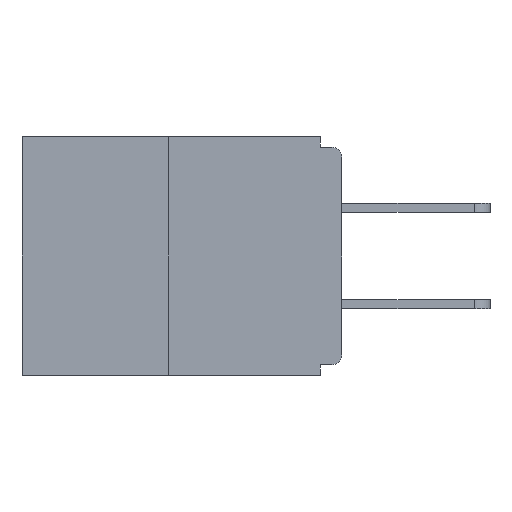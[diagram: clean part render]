
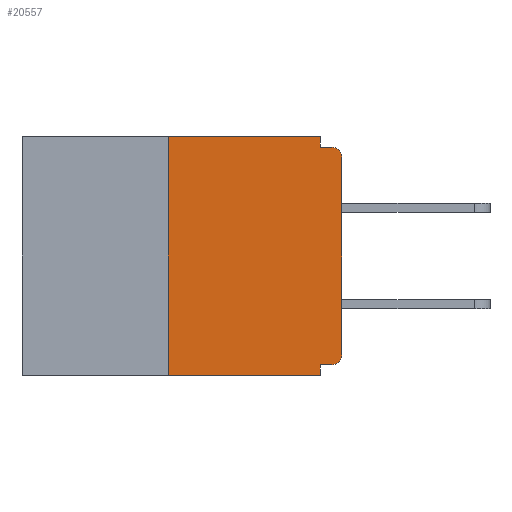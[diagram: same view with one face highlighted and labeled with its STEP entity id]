
A CAD part, left-side view. The second image highlights one B-rep face of the part: STEP entity #20557.
In plain terms, the highlighted planar face has unit normal (-1, 0, 0).
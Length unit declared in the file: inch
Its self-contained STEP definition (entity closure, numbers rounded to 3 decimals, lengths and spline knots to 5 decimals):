
#82 = CARTESIAN_POINT ( 'NONE',  ( 0., 0., -0.313 ) ) ;
#915 = CARTESIAN_POINT ( 'NONE',  ( 0., 0.031, -0.343 ) ) ;
#980 = FACE_OUTER_BOUND ( 'NONE', #16924, .T. ) ;
#1281 = AXIS2_PLACEMENT_3D ( 'NONE', #12804, #26548, #19624 ) ;
#1932 = ORIENTED_EDGE ( 'NONE', *, *, #6291, .F. ) ;
#2231 = DIRECTION ( 'NONE',  ( 0., 1., 0. ) ) ;
#2313 = VECTOR ( 'NONE', #6157, 39.37008 ) ;
#2456 = CARTESIAN_POINT ( 'NONE',  ( 0., 0.031, 0. ) ) ;
#3242 = ORIENTED_EDGE ( 'NONE', *, *, #16820, .T. ) ;
#4316 = AXIS2_PLACEMENT_3D ( 'NONE', #22192, #22400, #24754 ) ;
#4374 = CARTESIAN_POINT ( 'NONE',  ( 0., 0., -0.328 ) ) ;
#4790 = CARTESIAN_POINT ( 'NONE',  ( 0., 0.46, -0.343 ) ) ;
#5185 = VECTOR ( 'NONE', #20942, 39.37008 ) ;
#5370 = DIRECTION ( 'NONE',  ( -1., 0., 0. ) ) ;
#5688 = PLANE ( 'NONE',  #1281 ) ;
#5932 = CARTESIAN_POINT ( 'NONE',  ( 0., 0.015, -0.328 ) ) ;
#6157 = DIRECTION ( 'NONE',  ( 0., -1., 0. ) ) ;
#6177 = VERTEX_POINT ( 'NONE', #13023 ) ;
#6291 = EDGE_CURVE ( 'NONE', #12148, #25669, #15479, .T. ) ;
#6300 = VECTOR ( 'NONE', #26960, 39.37008 ) ;
#6679 = DIRECTION ( 'NONE',  ( 0., 0., -1. ) ) ;
#7107 = VERTEX_POINT ( 'NONE', #26876 ) ;
#8392 = VERTEX_POINT ( 'NONE', #5932 ) ;
#8402 = LINE ( 'NONE', #10453, #2313 ) ;
#9014 = DIRECTION ( 'NONE',  ( 0., 0., 1. ) ) ;
#9048 = VERTEX_POINT ( 'NONE', #23459 ) ;
#9910 = EDGE_CURVE ( 'NONE', #6177, #9048, #17129, .T. ) ;
#10453 = CARTESIAN_POINT ( 'NONE',  ( 0., 0., -0.015 ) ) ;
#11219 = DIRECTION ( 'NONE',  ( 0., 0., -1. ) ) ;
#11706 = VECTOR ( 'NONE', #25645, 39.37008 ) ;
#12148 = VERTEX_POINT ( 'NONE', #2456 ) ;
#12328 = DIRECTION ( 'NONE',  ( 0., 0., -1. ) ) ;
#12804 = CARTESIAN_POINT ( 'NONE',  ( 0., 0.46, 0. ) ) ;
#12903 = ORIENTED_EDGE ( 'NONE', *, *, #23056, .F. ) ;
#13023 = CARTESIAN_POINT ( 'NONE',  ( 0., 0., -0.03 ) ) ;
#13352 = ORIENTED_EDGE ( 'NONE', *, *, #15543, .F. ) ;
#13410 = CARTESIAN_POINT ( 'NONE',  ( 0., 0.031, -0.343 ) ) ;
#13500 = ORIENTED_EDGE ( 'NONE', *, *, #9910, .T. ) ;
#13683 = EDGE_CURVE ( 'NONE', #20784, #6177, #24740, .T. ) ;
#15479 = LINE ( 'NONE', #16085, #28198 ) ;
#15543 = EDGE_CURVE ( 'NONE', #8392, #7107, #28245, .T. ) ;
#16085 = CARTESIAN_POINT ( 'NONE',  ( 0., 0.031, 0. ) ) ;
#16293 = CARTESIAN_POINT ( 'NONE',  ( 0., 0.46, 0. ) ) ;
#16820 = EDGE_CURVE ( 'NONE', #8392, #20784, #22680, .T. ) ;
#16924 = EDGE_LOOP ( 'NONE', ( #20365, #18635, #19635, #12903, #13352, #3242, #23591, #13500, #29253, #1932 ) ) ;
#17129 = CIRCLE ( 'NONE', #22746, 0.015 ) ;
#17466 = LINE ( 'NONE', #16293, #5185 ) ;
#17514 = CARTESIAN_POINT ( 'NONE',  ( 0., 0., 0. ) ) ;
#18055 = VECTOR ( 'NONE', #9014, 39.37008 ) ;
#18635 = ORIENTED_EDGE ( 'NONE', *, *, #25573, .F. ) ;
#19084 = EDGE_CURVE ( 'NONE', #25669, #9048, #8402, .T. ) ;
#19191 = CARTESIAN_POINT ( 'NONE',  ( 0., 0.25, 0. ) ) ;
#19624 = DIRECTION ( 'NONE',  ( 0., 0., -1. ) ) ;
#19635 = ORIENTED_EDGE ( 'NONE', *, *, #22704, .T. ) ;
#19918 = VERTEX_POINT ( 'NONE', #23455 ) ;
#20365 = ORIENTED_EDGE ( 'NONE', *, *, #23443, .F. ) ;
#20557 = ADVANCED_FACE ( 'NONE', ( #980 ), #5688, .F. ) ;
#20683 = CARTESIAN_POINT ( 'NONE',  ( 0., 0.031, -0.015 ) ) ;
#20784 = VERTEX_POINT ( 'NONE', #82 ) ;
#20942 = DIRECTION ( 'NONE',  ( 0., -1., 0. ) ) ;
#21065 = VERTEX_POINT ( 'NONE', #19191 ) ;
#22017 = VECTOR ( 'NONE', #2231, 39.37008 ) ;
#22192 = CARTESIAN_POINT ( 'NONE',  ( 0., 0.015, -0.313 ) ) ;
#22400 = DIRECTION ( 'NONE',  ( -1., 0., 0. ) ) ;
#22680 = CIRCLE ( 'NONE', #4316, 0.015 ) ;
#22704 = EDGE_CURVE ( 'NONE', #19918, #22780, #26250, .T. ) ;
#22746 = AXIS2_PLACEMENT_3D ( 'NONE', #26146, #5370, #12328 ) ;
#22780 = VERTEX_POINT ( 'NONE', #915 ) ;
#22889 = CARTESIAN_POINT ( 'NONE',  ( 0., 0.25, 0. ) ) ;
#23056 = EDGE_CURVE ( 'NONE', #7107, #22780, #29829, .T. ) ;
#23443 = EDGE_CURVE ( 'NONE', #21065, #12148, #17466, .T. ) ;
#23455 = CARTESIAN_POINT ( 'NONE',  ( 0., 0.25, -0.343 ) ) ;
#23459 = CARTESIAN_POINT ( 'NONE',  ( 0., 0.015, -0.015 ) ) ;
#23591 = ORIENTED_EDGE ( 'NONE', *, *, #13683, .T. ) ;
#24200 = LINE ( 'NONE', #22889, #18055 ) ;
#24740 = LINE ( 'NONE', #17514, #6300 ) ;
#24754 = DIRECTION ( 'NONE',  ( 0., 0., -1. ) ) ;
#25573 = EDGE_CURVE ( 'NONE', #19918, #21065, #24200, .T. ) ;
#25645 = DIRECTION ( 'NONE',  ( 0., -1., 0. ) ) ;
#25669 = VERTEX_POINT ( 'NONE', #20683 ) ;
#26146 = CARTESIAN_POINT ( 'NONE',  ( 0., 0.015, -0.03 ) ) ;
#26250 = LINE ( 'NONE', #4790, #11706 ) ;
#26548 = DIRECTION ( 'NONE',  ( 1., 0., 0. ) ) ;
#26876 = CARTESIAN_POINT ( 'NONE',  ( 0., 0.031, -0.328 ) ) ;
#26960 = DIRECTION ( 'NONE',  ( 0., 0., 1. ) ) ;
#28198 = VECTOR ( 'NONE', #11219, 39.37008 ) ;
#28245 = LINE ( 'NONE', #4374, #22017 ) ;
#29253 = ORIENTED_EDGE ( 'NONE', *, *, #19084, .F. ) ;
#29454 = VECTOR ( 'NONE', #6679, 39.37008 ) ;
#29829 = LINE ( 'NONE', #13410, #29454 ) ;
